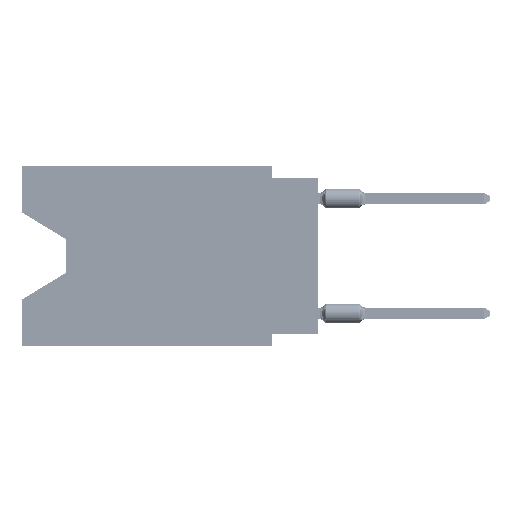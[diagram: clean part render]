
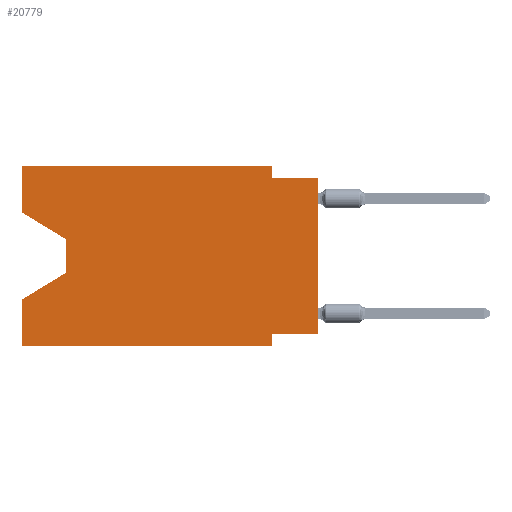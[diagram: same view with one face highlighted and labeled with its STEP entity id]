
A CAD part, left-side view. The second image highlights one B-rep face of the part: STEP entity #20779.
In plain terms, the highlighted planar face has unit normal (-1, 0, 0).
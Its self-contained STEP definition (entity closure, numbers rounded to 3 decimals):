
#1824 = CARTESIAN_POINT ( 'NONE',  ( 0., 2.54, 0. ) ) ;
#2230 = VERTEX_POINT ( 'NONE', #47919 ) ;
#2902 = EDGE_CURVE ( 'NONE', #34384, #2230, #80009, .T. ) ;
#3984 = VECTOR ( 'NONE', #39839, 1000. ) ;
#4508 = ORIENTED_EDGE ( 'NONE', *, *, #17356, .F. ) ;
#5163 = VECTOR ( 'NONE', #42110, 1000. ) ;
#5218 = VECTOR ( 'NONE', #33982, 1000. ) ;
#6196 = EDGE_CURVE ( 'NONE', #34384, #28767, #55192, .T. ) ;
#6209 = CARTESIAN_POINT ( 'NONE',  ( 0., 0., 0. ) ) ;
#6559 = DIRECTION ( 'NONE',  ( 0., -0.855, -0.519 ) ) ;
#7809 = ORIENTED_EDGE ( 'NONE', *, *, #6196, .T. ) ;
#7829 = CARTESIAN_POINT ( 'NONE',  ( 0., 0., -9.271 ) ) ;
#8208 = VECTOR ( 'NONE', #56704, 1000. ) ;
#8431 = ORIENTED_EDGE ( 'NONE', *, *, #15869, .F. ) ;
#11047 = VERTEX_POINT ( 'NONE', #12207 ) ;
#11370 = PLANE ( 'NONE',  #18679 ) ;
#11500 = VERTEX_POINT ( 'NONE', #38985 ) ;
#11558 = ORIENTED_EDGE ( 'NONE', *, *, #32692, .T. ) ;
#11828 = VECTOR ( 'NONE', #6559, 1000. ) ;
#12207 = CARTESIAN_POINT ( 'NONE',  ( 0., 13.97, -5.893 ) ) ;
#12867 = CARTESIAN_POINT ( 'NONE',  ( 0., 16.383, -9.906 ) ) ;
#14181 = DIRECTION ( 'NONE',  ( 0., -1., 0. ) ) ;
#14620 = CARTESIAN_POINT ( 'NONE',  ( 0., 16.383, 0. ) ) ;
#14637 = DIRECTION ( 'NONE',  ( 0., 0., 1. ) ) ;
#15869 = EDGE_CURVE ( 'NONE', #53652, #28767, #82241, .T. ) ;
#16034 = DIRECTION ( 'NONE',  ( 0., 0.855, -0.519 ) ) ;
#16133 = ORIENTED_EDGE ( 'NONE', *, *, #38365, .T. ) ;
#16172 = CARTESIAN_POINT ( 'NONE',  ( 0., 0., -0.635 ) ) ;
#16491 = EDGE_CURVE ( 'NONE', #16939, #53652, #57453, .T. ) ;
#16939 = VERTEX_POINT ( 'NONE', #83536 ) ;
#17356 = EDGE_CURVE ( 'NONE', #71474, #45577, #62885, .T. ) ;
#18679 = AXIS2_PLACEMENT_3D ( 'NONE', #25023, #52800, #53262 ) ;
#20182 = VERTEX_POINT ( 'NONE', #61024 ) ;
#20229 = LINE ( 'NONE', #68533, #3984 ) ;
#20779 = ADVANCED_FACE ( 'NONE', ( #47323 ), #11370, .F. ) ;
#21305 = CARTESIAN_POINT ( 'NONE',  ( 0., 2.54, -0.635 ) ) ;
#21535 = CARTESIAN_POINT ( 'NONE',  ( 0., 2.54, -9.906 ) ) ;
#23119 = EDGE_CURVE ( 'NONE', #11500, #71474, #77045, .T. ) ;
#25023 = CARTESIAN_POINT ( 'NONE',  ( 0., 16.383, 0. ) ) ;
#25682 = VECTOR ( 'NONE', #16034, 1000. ) ;
#26689 = LINE ( 'NONE', #6209, #5218 ) ;
#28238 = CARTESIAN_POINT ( 'NONE',  ( 0., 2.54, -9.271 ) ) ;
#28557 = VECTOR ( 'NONE', #50170, 1000. ) ;
#28767 = VERTEX_POINT ( 'NONE', #21535 ) ;
#29121 = EDGE_CURVE ( 'NONE', #45577, #64181, #63321, .T. ) ;
#32692 = EDGE_CURVE ( 'NONE', #11500, #20182, #48893, .T. ) ;
#33982 = DIRECTION ( 'NONE',  ( 0., 0., 1. ) ) ;
#34384 = VERTEX_POINT ( 'NONE', #63354 ) ;
#36087 = VECTOR ( 'NONE', #67535, 1000. ) ;
#37145 = VECTOR ( 'NONE', #44462, 1000. ) ;
#38365 = EDGE_CURVE ( 'NONE', #16939, #46798, #26689, .T. ) ;
#38985 = CARTESIAN_POINT ( 'NONE',  ( 0., 16.383, -2.546 ) ) ;
#39839 = DIRECTION ( 'NONE',  ( 0., 0., -1. ) ) ;
#40008 = EDGE_CURVE ( 'NONE', #20182, #11047, #20229, .T. ) ;
#42110 = DIRECTION ( 'NONE',  ( 0., 0., -1. ) ) ;
#43671 = ORIENTED_EDGE ( 'NONE', *, *, #2902, .F. ) ;
#44462 = DIRECTION ( 'NONE',  ( 0., 0., 1. ) ) ;
#45577 = VERTEX_POINT ( 'NONE', #61983 ) ;
#46798 = VERTEX_POINT ( 'NONE', #53371 ) ;
#47323 = FACE_OUTER_BOUND ( 'NONE', #72260, .T. ) ;
#47919 = CARTESIAN_POINT ( 'NONE',  ( 0., 16.383, -7.36 ) ) ;
#48893 = LINE ( 'NONE', #83096, #11828 ) ;
#50170 = DIRECTION ( 'NONE',  ( 0., 1., 0. ) ) ;
#50364 = ORIENTED_EDGE ( 'NONE', *, *, #54044, .F. ) ;
#51713 = VECTOR ( 'NONE', #14181, 1000. ) ;
#52478 = ORIENTED_EDGE ( 'NONE', *, *, #29121, .F. ) ;
#52557 = ORIENTED_EDGE ( 'NONE', *, *, #83304, .T. ) ;
#52800 = DIRECTION ( 'NONE',  ( 1., 0., 0. ) ) ;
#53262 = DIRECTION ( 'NONE',  ( 0., 0., -1. ) ) ;
#53371 = CARTESIAN_POINT ( 'NONE',  ( 0., 0., -0.635 ) ) ;
#53652 = VERTEX_POINT ( 'NONE', #28238 ) ;
#54044 = EDGE_CURVE ( 'NONE', #64181, #46798, #58061, .T. ) ;
#55192 = LINE ( 'NONE', #12867, #36087 ) ;
#55206 = CARTESIAN_POINT ( 'NONE',  ( 0., 16.383, 0. ) ) ;
#56704 = DIRECTION ( 'NONE',  ( 0., -1., 0. ) ) ;
#56928 = DIRECTION ( 'NONE',  ( 0., 0., -1. ) ) ;
#57453 = LINE ( 'NONE', #7829, #28557 ) ;
#57464 = LINE ( 'NONE', #85293, #25682 ) ;
#58061 = LINE ( 'NONE', #16172, #8208 ) ;
#61024 = CARTESIAN_POINT ( 'NONE',  ( 0., 13.97, -4.013 ) ) ;
#61707 = CARTESIAN_POINT ( 'NONE',  ( 0., 2.54, -9.906 ) ) ;
#61983 = CARTESIAN_POINT ( 'NONE',  ( 0., 2.54, 0. ) ) ;
#62885 = LINE ( 'NONE', #14620, #51713 ) ;
#63321 = LINE ( 'NONE', #1824, #65421 ) ;
#63354 = CARTESIAN_POINT ( 'NONE',  ( 0., 16.383, -9.906 ) ) ;
#64181 = VERTEX_POINT ( 'NONE', #21305 ) ;
#64712 = CARTESIAN_POINT ( 'NONE',  ( 0., 16.383, 0. ) ) ;
#65421 = VECTOR ( 'NONE', #56928, 1000. ) ;
#66767 = CARTESIAN_POINT ( 'NONE',  ( 0., 16.383, 0. ) ) ;
#67535 = DIRECTION ( 'NONE',  ( 0., -1., 0. ) ) ;
#68533 = CARTESIAN_POINT ( 'NONE',  ( 0., 13.97, -4.013 ) ) ;
#71474 = VERTEX_POINT ( 'NONE', #55206 ) ;
#72260 = EDGE_LOOP ( 'NONE', ( #11558, #75975, #52557, #43671, #7809, #8431, #87910, #16133, #50364, #52478, #4508, #78561 ) ) ;
#73007 = VECTOR ( 'NONE', #14637, 1000. ) ;
#75975 = ORIENTED_EDGE ( 'NONE', *, *, #40008, .T. ) ;
#77045 = LINE ( 'NONE', #64712, #73007 ) ;
#78561 = ORIENTED_EDGE ( 'NONE', *, *, #23119, .F. ) ;
#80009 = LINE ( 'NONE', #66767, #37145 ) ;
#82241 = LINE ( 'NONE', #61707, #5163 ) ;
#83096 = CARTESIAN_POINT ( 'NONE',  ( 0., 16.383, -2.546 ) ) ;
#83304 = EDGE_CURVE ( 'NONE', #11047, #2230, #57464, .T. ) ;
#83536 = CARTESIAN_POINT ( 'NONE',  ( 0., 0., -9.271 ) ) ;
#85293 = CARTESIAN_POINT ( 'NONE',  ( 0., 13.97, -5.893 ) ) ;
#87910 = ORIENTED_EDGE ( 'NONE', *, *, #16491, .F. ) ;
